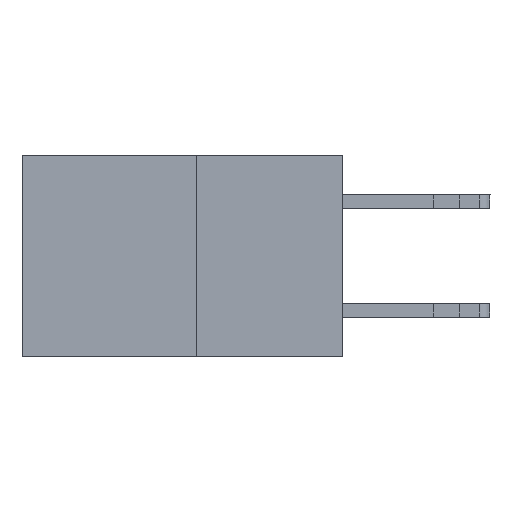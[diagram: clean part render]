
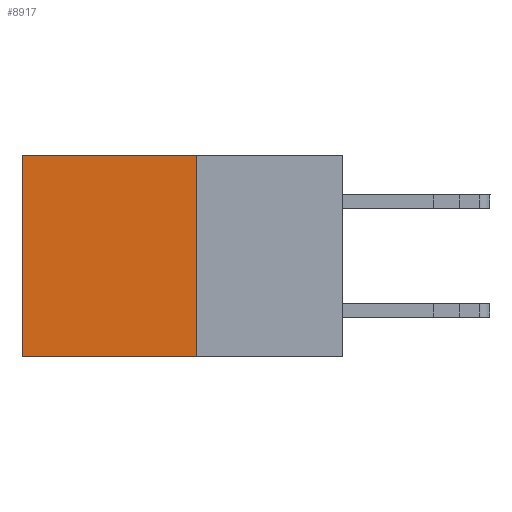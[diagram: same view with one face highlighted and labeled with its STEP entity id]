
A CAD part, left-side view. The second image highlights one B-rep face of the part: STEP entity #8917.
In plain terms, the highlighted planar face has unit normal (-1, 0, 0).
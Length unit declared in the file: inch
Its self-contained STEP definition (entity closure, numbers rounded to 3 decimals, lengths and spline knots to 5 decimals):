
#1162 = CARTESIAN_POINT ( 'NONE',  ( 0.277, 0.59, -0.37 ) ) ;
#1486 = DIRECTION ( 'NONE',  ( 0., 0., -1. ) ) ;
#1604 = EDGE_CURVE ( 'NONE', #3798, #14883, #3573, .T. ) ;
#1954 = ORIENTED_EDGE ( 'NONE', *, *, #12670, .F. ) ;
#2374 = VERTEX_POINT ( 'NONE', #9261 ) ;
#3202 = VECTOR ( 'NONE', #14080, 39.37008 ) ;
#3573 = LINE ( 'NONE', #8073, #14979 ) ;
#3706 = ORIENTED_EDGE ( 'NONE', *, *, #1604, .F. ) ;
#3798 = VERTEX_POINT ( 'NONE', #12131 ) ;
#4724 = VECTOR ( 'NONE', #11447, 39.37008 ) ;
#4900 = VECTOR ( 'NONE', #1486, 39.37008 ) ;
#4916 = AXIS2_PLACEMENT_3D ( 'NONE', #6009, #11933, #6077 ) ;
#4986 = LINE ( 'NONE', #11922, #4900 ) ;
#5725 = LINE ( 'NONE', #1162, #4724 ) ;
#6009 = CARTESIAN_POINT ( 'NONE',  ( 0.277, 0.27, -0.37 ) ) ;
#6077 = DIRECTION ( 'NONE',  ( 0., 0., -1. ) ) ;
#6632 = FACE_OUTER_BOUND ( 'NONE', #9743, .T. ) ;
#7688 = ORIENTED_EDGE ( 'NONE', *, *, #14494, .T. ) ;
#8004 = EDGE_CURVE ( 'NONE', #2374, #12946, #8250, .T. ) ;
#8073 = CARTESIAN_POINT ( 'NONE',  ( 0.277, 0.27, -0.37 ) ) ;
#8229 = DIRECTION ( 'NONE',  ( 0., 1., 0. ) ) ;
#8250 = LINE ( 'NONE', #14237, #3202 ) ;
#8917 = ADVANCED_FACE ( 'NONE', ( #6632 ), #11870, .F. ) ;
#8976 = CARTESIAN_POINT ( 'NONE',  ( 0.277, 0.59, -0.37 ) ) ;
#9261 = CARTESIAN_POINT ( 'NONE',  ( 0.277, 0.27, 0. ) ) ;
#9743 = EDGE_LOOP ( 'NONE', ( #7688, #3706, #1954, #14912 ) ) ;
#10243 = CARTESIAN_POINT ( 'NONE',  ( 0.277, 0.59, 0. ) ) ;
#11447 = DIRECTION ( 'NONE',  ( 0., 0., -1. ) ) ;
#11870 = PLANE ( 'NONE',  #4916 ) ;
#11922 = CARTESIAN_POINT ( 'NONE',  ( 0.277, 0.27, -0.37 ) ) ;
#11933 = DIRECTION ( 'NONE',  ( 1., 0., 0. ) ) ;
#12131 = CARTESIAN_POINT ( 'NONE',  ( 0.277, 0.27, -0.37 ) ) ;
#12670 = EDGE_CURVE ( 'NONE', #2374, #3798, #4986, .T. ) ;
#12946 = VERTEX_POINT ( 'NONE', #10243 ) ;
#14080 = DIRECTION ( 'NONE',  ( 0., 1., 0. ) ) ;
#14237 = CARTESIAN_POINT ( 'NONE',  ( 0.277, 0.27, 0. ) ) ;
#14494 = EDGE_CURVE ( 'NONE', #12946, #14883, #5725, .T. ) ;
#14883 = VERTEX_POINT ( 'NONE', #8976 ) ;
#14912 = ORIENTED_EDGE ( 'NONE', *, *, #8004, .T. ) ;
#14979 = VECTOR ( 'NONE', #8229, 39.37008 ) ;
